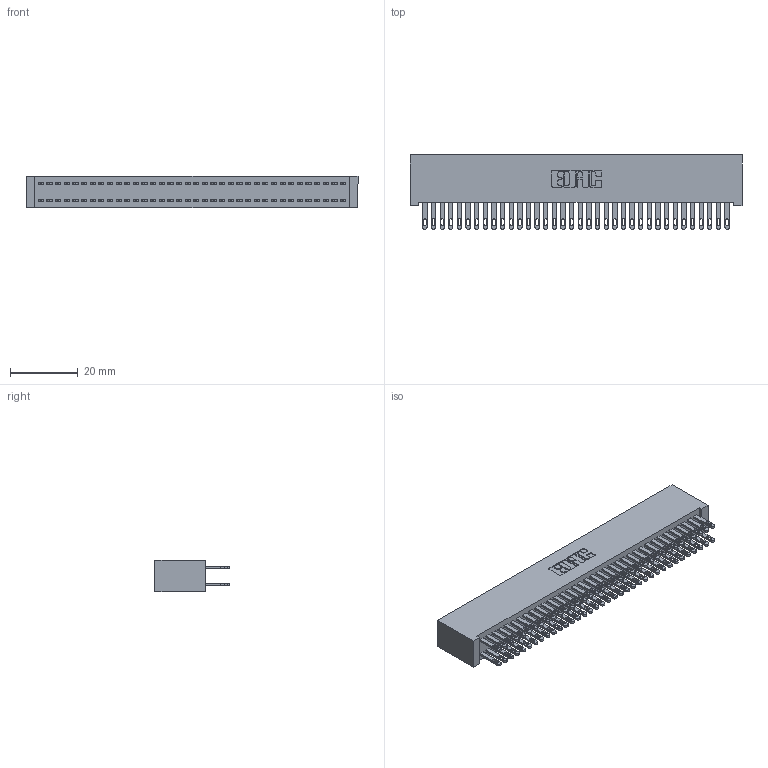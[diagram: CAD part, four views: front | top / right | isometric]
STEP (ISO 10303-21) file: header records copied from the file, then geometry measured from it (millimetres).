
FILE_DESCRIPTION (( 'STEP AP203' ), '1' );
FILE_NAME ('892-072-500-201.STEP', '2020-09-21T19:43:52', ( '' ), ( '' ), 'SwSTEP 2.0', 'SolidWorks 2020', '' );
FILE_SCHEMA (( 'CONFIG_CONTROL_DESIGN' ));
Length unit declared in the file: inch
Products named in the file (3): 842 Part_Lugless; 345-292-001_345-293-100; 892-072-500-201
Assembly tree (73 placements, depth 2):
  892-072-500-201
    842 Part_Lugless
    345-292-001_345-293-100  x72
Bounding box: 97.69 x 21.85 x 9.4 mm (x, y, z)
Volume: 9408.4 mm3; surface area: 16302.3 mm2
Topology: 73 solids, 73 shells, 3558 faces, 10859 edges, 7238 vertices
Faces by surface type: plane 2222, cylinder 1336
Entity records: 23457 total; most frequent: CARTESIAN_POINT 3890, ORIENTED_EDGE 3826, DIRECTION 3329, EDGE_CURVE 1913, VECTOR 1789, LINE 1789, VERTEX_POINT 1274, AXIS2_PLACEMENT_3D 770
